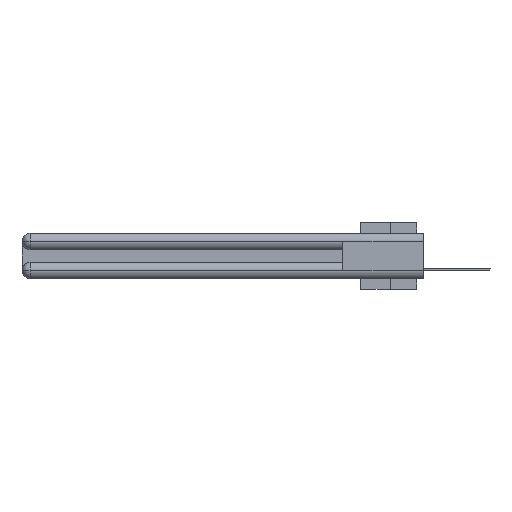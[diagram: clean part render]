
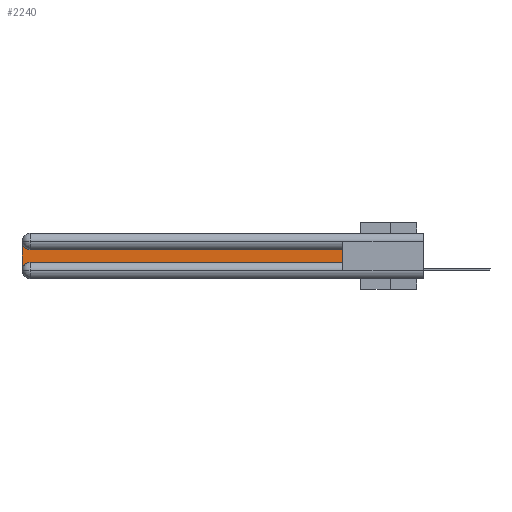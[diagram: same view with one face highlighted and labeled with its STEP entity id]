
A CAD part, left-side view. The second image highlights one B-rep face of the part: STEP entity #2240.
In plain terms, the highlighted planar face has unit normal (-1, 0, 0).
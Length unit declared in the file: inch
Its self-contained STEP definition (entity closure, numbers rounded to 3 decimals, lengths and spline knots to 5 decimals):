
#1527 = ORIENTED_EDGE ( 'NONE', *, *, #24362, .T. ) ;
#2240 = ADVANCED_FACE ( 'NONE', ( #12352 ), #30248, .F. ) ;
#3286 = AXIS2_PLACEMENT_3D ( 'NONE', #27423, #4567, #22464 ) ;
#3434 = CARTESIAN_POINT ( 'NONE',  ( 0.075, 0.6, -0.1225 ) ) ;
#3479 = CARTESIAN_POINT ( 'NONE',  ( 0.075, 2.94, -0.1225 ) ) ;
#3596 = VERTEX_POINT ( 'NONE', #9923 ) ;
#4567 = DIRECTION ( 'NONE',  ( 1., 0., 0. ) ) ;
#5137 = LINE ( 'NONE', #17895, #31445 ) ;
#5494 = CARTESIAN_POINT ( 'NONE',  ( 0.075, 0.6, -0.2175 ) ) ;
#7361 = DIRECTION ( 'NONE',  ( 1., 0., 0. ) ) ;
#7861 = CARTESIAN_POINT ( 'NONE',  ( 0.075, 2.94, -0.0625 ) ) ;
#9923 = CARTESIAN_POINT ( 'NONE',  ( 0.075, 0.6, -0.2175 ) ) ;
#9930 = EDGE_CURVE ( 'NONE', #18532, #3596, #20989, .T. ) ;
#10532 = ORIENTED_EDGE ( 'NONE', *, *, #28977, .T. ) ;
#11014 = VERTEX_POINT ( 'NONE', #11598 ) ;
#11598 = CARTESIAN_POINT ( 'NONE',  ( 0.075, 3., -0.0625 ) ) ;
#11813 = ORIENTED_EDGE ( 'NONE', *, *, #28484, .T. ) ;
#12352 = FACE_OUTER_BOUND ( 'NONE', #32018, .T. ) ;
#12722 = CIRCLE ( 'NONE', #15887, 0.06 ) ;
#13647 = ORIENTED_EDGE ( 'NONE', *, *, #28128, .T. ) ;
#13736 = VERTEX_POINT ( 'NONE', #3434 ) ;
#15280 = LINE ( 'NONE', #5494, #18716 ) ;
#15510 = DIRECTION ( 'NONE',  ( 0., -1., 0. ) ) ;
#15887 = AXIS2_PLACEMENT_3D ( 'NONE', #7861, #17975, #28079 ) ;
#15967 = VECTOR ( 'NONE', #15510, 39.37008 ) ;
#16131 = CARTESIAN_POINT ( 'NONE',  ( 0.075, 0.6, -0.1225 ) ) ;
#17895 = CARTESIAN_POINT ( 'NONE',  ( 0.075, 3., -0.2175 ) ) ;
#17975 = DIRECTION ( 'NONE',  ( 1., 0., 0. ) ) ;
#18022 = ORIENTED_EDGE ( 'NONE', *, *, #9930, .T. ) ;
#18133 = ORIENTED_EDGE ( 'NONE', *, *, #28736, .T. ) ;
#18532 = VERTEX_POINT ( 'NONE', #25698 ) ;
#18586 = VERTEX_POINT ( 'NONE', #3479 ) ;
#18716 = VECTOR ( 'NONE', #25382, 39.37008 ) ;
#19574 = CARTESIAN_POINT ( 'NONE',  ( 0.075, 3., -0.2775 ) ) ;
#19802 = CARTESIAN_POINT ( 'NONE',  ( 0.075, 2.94, -0.2775 ) ) ;
#20989 = LINE ( 'NONE', #22965, #15967 ) ;
#21372 = VERTEX_POINT ( 'NONE', #19574 ) ;
#22464 = DIRECTION ( 'NONE',  ( 0., 0., -1. ) ) ;
#22941 = LINE ( 'NONE', #16131, #30847 ) ;
#22965 = CARTESIAN_POINT ( 'NONE',  ( 0.075, 0.6, -0.2175 ) ) ;
#24031 = CIRCLE ( 'NONE', #32416, 0.06 ) ;
#24362 = EDGE_CURVE ( 'NONE', #18586, #11014, #12722, .T. ) ;
#25382 = DIRECTION ( 'NONE',  ( 0., 0., 1. ) ) ;
#25698 = CARTESIAN_POINT ( 'NONE',  ( 0.075, 2.94, -0.2175 ) ) ;
#26247 = DIRECTION ( 'NONE',  ( 0., 1., 0. ) ) ;
#27423 = CARTESIAN_POINT ( 'NONE',  ( 0.075, 3., -0.1225 ) ) ;
#28079 = DIRECTION ( 'NONE',  ( 0., 0., -1. ) ) ;
#28128 = EDGE_CURVE ( 'NONE', #3596, #13736, #15280, .T. ) ;
#28484 = EDGE_CURVE ( 'NONE', #11014, #21372, #5137, .T. ) ;
#28736 = EDGE_CURVE ( 'NONE', #21372, #18532, #24031, .T. ) ;
#28977 = EDGE_CURVE ( 'NONE', #13736, #18586, #22941, .T. ) ;
#30248 = PLANE ( 'NONE',  #3286 ) ;
#30847 = VECTOR ( 'NONE', #26247, 39.37008 ) ;
#31445 = VECTOR ( 'NONE', #32643, 39.37008 ) ;
#32018 = EDGE_LOOP ( 'NONE', ( #10532, #1527, #11813, #18133, #18022, #13647 ) ) ;
#32375 = DIRECTION ( 'NONE',  ( 0., 0., -1. ) ) ;
#32416 = AXIS2_PLACEMENT_3D ( 'NONE', #19802, #7361, #32375 ) ;
#32643 = DIRECTION ( 'NONE',  ( 0., 0., -1. ) ) ;
